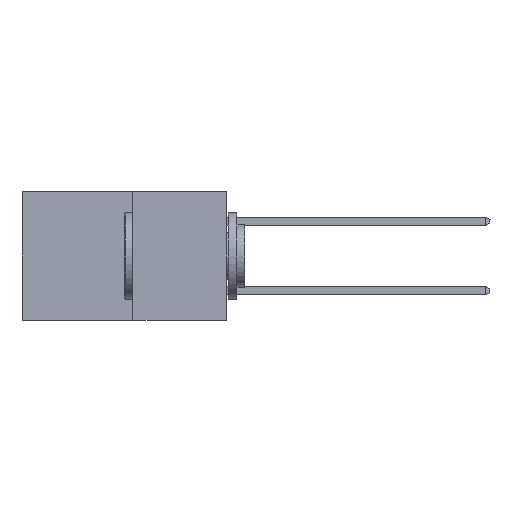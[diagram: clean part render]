
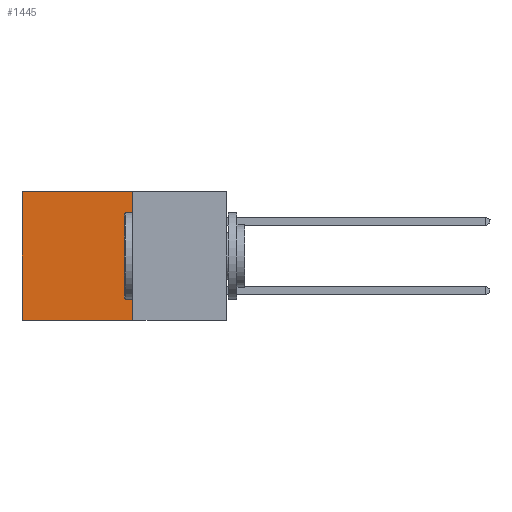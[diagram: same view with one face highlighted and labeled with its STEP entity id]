
A CAD part, left-side view. The second image highlights one B-rep face of the part: STEP entity #1445.
In plain terms, the highlighted planar face has unit normal (-1, 0, 0).
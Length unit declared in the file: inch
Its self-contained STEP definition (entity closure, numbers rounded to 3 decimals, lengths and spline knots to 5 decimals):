
#196 = DIRECTION ( 'NONE',  ( 0., 0., -1. ) ) ;
#1445 = ADVANCED_FACE ( 'NONE', ( #13410 ), #7424, .F. ) ;
#1520 = CARTESIAN_POINT ( 'NONE',  ( 0.277, 0.27, -0.37 ) ) ;
#2152 = VECTOR ( 'NONE', #6191, 39.37008 ) ;
#2256 = EDGE_CURVE ( 'NONE', #15967, #18957, #16006, .T. ) ;
#2347 = EDGE_CURVE ( 'NONE', #17785, #15967, #11000, .T. ) ;
#3755 = ORIENTED_EDGE ( 'NONE', *, *, #18876, .T. ) ;
#3859 = VECTOR ( 'NONE', #19187, 39.37008 ) ;
#4077 = AXIS2_PLACEMENT_3D ( 'NONE', #11725, #8096, #13012 ) ;
#4249 = ORIENTED_EDGE ( 'NONE', *, *, #17196, .T. ) ;
#4901 = CARTESIAN_POINT ( 'NONE',  ( 0.277, 0.27, 0. ) ) ;
#5022 = CARTESIAN_POINT ( 'NONE',  ( 0.277, 0.27, 0. ) ) ;
#6191 = DIRECTION ( 'NONE',  ( 0., 0., -1. ) ) ;
#6298 = LINE ( 'NONE', #10816, #2152 ) ;
#6388 = VECTOR ( 'NONE', #196, 39.37008 ) ;
#6488 = DIRECTION ( 'NONE',  ( 0., 1., 0. ) ) ;
#7424 = PLANE ( 'NONE',  #4077 ) ;
#7934 = ORIENTED_EDGE ( 'NONE', *, *, #2256, .F. ) ;
#8096 = DIRECTION ( 'NONE',  ( 1., 0., 0. ) ) ;
#8599 = EDGE_LOOP ( 'NONE', ( #3755, #7934, #12069, #4249 ) ) ;
#10740 = CARTESIAN_POINT ( 'NONE',  ( 0.277, 0.59, 0. ) ) ;
#10816 = CARTESIAN_POINT ( 'NONE',  ( 0.277, 0.59, -0.37 ) ) ;
#11000 = LINE ( 'NONE', #1520, #6388 ) ;
#11015 = CARTESIAN_POINT ( 'NONE',  ( 0.277, 0.59, -0.37 ) ) ;
#11191 = VERTEX_POINT ( 'NONE', #10740 ) ;
#11725 = CARTESIAN_POINT ( 'NONE',  ( 0.277, 0.27, -0.37 ) ) ;
#12069 = ORIENTED_EDGE ( 'NONE', *, *, #2347, .F. ) ;
#12711 = LINE ( 'NONE', #4901, #17687 ) ;
#13012 = DIRECTION ( 'NONE',  ( 0., 0., -1. ) ) ;
#13410 = FACE_OUTER_BOUND ( 'NONE', #8599, .T. ) ;
#15967 = VERTEX_POINT ( 'NONE', #17454 ) ;
#16006 = LINE ( 'NONE', #19590, #3859 ) ;
#17196 = EDGE_CURVE ( 'NONE', #17785, #11191, #12711, .T. ) ;
#17454 = CARTESIAN_POINT ( 'NONE',  ( 0.277, 0.27, -0.37 ) ) ;
#17687 = VECTOR ( 'NONE', #6488, 39.37008 ) ;
#17785 = VERTEX_POINT ( 'NONE', #5022 ) ;
#18876 = EDGE_CURVE ( 'NONE', #11191, #18957, #6298, .T. ) ;
#18957 = VERTEX_POINT ( 'NONE', #11015 ) ;
#19187 = DIRECTION ( 'NONE',  ( 0., 1., 0. ) ) ;
#19590 = CARTESIAN_POINT ( 'NONE',  ( 0.277, 0.27, -0.37 ) ) ;
